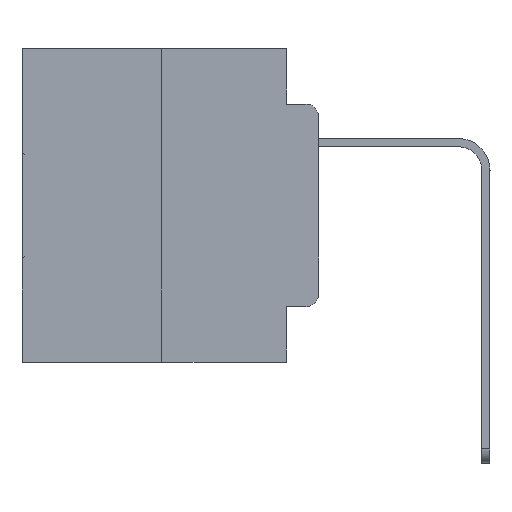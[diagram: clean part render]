
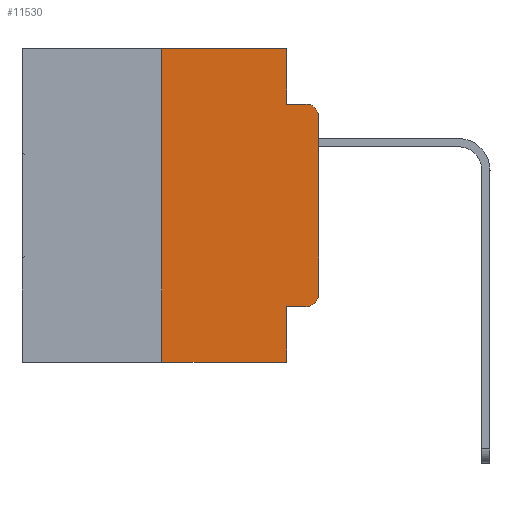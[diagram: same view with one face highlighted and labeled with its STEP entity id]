
A CAD part, left-side view. The second image highlights one B-rep face of the part: STEP entity #11530.
In plain terms, the highlighted planar face has unit normal (-1, 0, 0).
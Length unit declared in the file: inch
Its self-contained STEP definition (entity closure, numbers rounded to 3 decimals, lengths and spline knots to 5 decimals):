
#555 = DIRECTION ( 'NONE',  ( -1., 0., 0. ) ) ;
#612 = ORIENTED_EDGE ( 'NONE', *, *, #26887, .F. ) ;
#956 = CARTESIAN_POINT ( 'NONE',  ( 0., 0.02, -0.4115 ) ) ;
#1612 = LINE ( 'NONE', #6026, #26392 ) ;
#1768 = ORIENTED_EDGE ( 'NONE', *, *, #15779, .T. ) ;
#1941 = VERTEX_POINT ( 'NONE', #22275 ) ;
#2228 = DIRECTION ( 'NONE',  ( -1., 0., 0. ) ) ;
#2858 = CARTESIAN_POINT ( 'NONE',  ( 0., 0.02, -0.3915 ) ) ;
#3165 = DIRECTION ( 'NONE',  ( 0., 0., -1. ) ) ;
#3425 = VECTOR ( 'NONE', #10558, 39.37008 ) ;
#3594 = VERTEX_POINT ( 'NONE', #9480 ) ;
#3764 = DIRECTION ( 'NONE',  ( 0., -1., 0. ) ) ;
#3897 = EDGE_CURVE ( 'NONE', #1941, #20254, #21566, .T. ) ;
#3945 = EDGE_CURVE ( 'NONE', #5392, #29817, #1612, .T. ) ;
#4189 = ORIENTED_EDGE ( 'NONE', *, *, #19723, .T. ) ;
#5392 = VERTEX_POINT ( 'NONE', #6243 ) ;
#5624 = DIRECTION ( 'NONE',  ( 0., -1., 0. ) ) ;
#5630 = LINE ( 'NONE', #12832, #3425 ) ;
#6026 = CARTESIAN_POINT ( 'NONE',  ( 0., 0., 0. ) ) ;
#6243 = CARTESIAN_POINT ( 'NONE',  ( 0., 0., -0.3915 ) ) ;
#6244 = CARTESIAN_POINT ( 'NONE',  ( 0., 0.25, 0. ) ) ;
#7311 = CARTESIAN_POINT ( 'NONE',  ( 0., 0.02, -0.0885 ) ) ;
#8079 = VERTEX_POINT ( 'NONE', #20498 ) ;
#8158 = CARTESIAN_POINT ( 'NONE',  ( 0., 0.051, -0.5 ) ) ;
#8228 = LINE ( 'NONE', #28824, #13765 ) ;
#8421 = VERTEX_POINT ( 'NONE', #7311 ) ;
#9480 = CARTESIAN_POINT ( 'NONE',  ( 0., 0.051, -0.0885 ) ) ;
#10358 = VERTEX_POINT ( 'NONE', #956 ) ;
#10513 = DIRECTION ( 'NONE',  ( 1., 0., 0. ) ) ;
#10558 = DIRECTION ( 'NONE',  ( 0., 0., -1. ) ) ;
#11530 = ADVANCED_FACE ( 'NONE', ( #17773 ), #19885, .F. ) ;
#12347 = ORIENTED_EDGE ( 'NONE', *, *, #20374, .F. ) ;
#12472 = DIRECTION ( 'NONE',  ( 0., -1., 0. ) ) ;
#12832 = CARTESIAN_POINT ( 'NONE',  ( 0., 0.051, 0. ) ) ;
#13064 = LINE ( 'NONE', #17302, #20425 ) ;
#13093 = DIRECTION ( 'NONE',  ( 0., 0., -1. ) ) ;
#13266 = LINE ( 'NONE', #6244, #18780 ) ;
#13474 = DIRECTION ( 'NONE',  ( 0., 0., 1. ) ) ;
#13765 = VECTOR ( 'NONE', #12472, 39.37008 ) ;
#14086 = ORIENTED_EDGE ( 'NONE', *, *, #17543, .T. ) ;
#14752 = DIRECTION ( 'NONE',  ( 0., 0., -1. ) ) ;
#15779 = EDGE_CURVE ( 'NONE', #27083, #28043, #29642, .T. ) ;
#15990 = ORIENTED_EDGE ( 'NONE', *, *, #3897, .F. ) ;
#16454 = CIRCLE ( 'NONE', #26101, 0.02 ) ;
#16767 = CARTESIAN_POINT ( 'NONE',  ( 0., 0.25, -0.5 ) ) ;
#17117 = DIRECTION ( 'NONE',  ( 0., -1., 0. ) ) ;
#17302 = CARTESIAN_POINT ( 'NONE',  ( 0., 0.051, 0. ) ) ;
#17543 = EDGE_CURVE ( 'NONE', #8079, #10358, #19461, .T. ) ;
#17773 = FACE_OUTER_BOUND ( 'NONE', #30167, .T. ) ;
#18365 = VECTOR ( 'NONE', #17117, 39.37008 ) ;
#18780 = VECTOR ( 'NONE', #13474, 39.37008 ) ;
#19461 = LINE ( 'NONE', #28915, #18365 ) ;
#19723 = EDGE_CURVE ( 'NONE', #29817, #8421, #16454, .T. ) ;
#19770 = ORIENTED_EDGE ( 'NONE', *, *, #26565, .T. ) ;
#19861 = VECTOR ( 'NONE', #3764, 39.37008 ) ;
#19885 = PLANE ( 'NONE',  #29152 ) ;
#20029 = CARTESIAN_POINT ( 'NONE',  ( 0., 0.473, -0.5 ) ) ;
#20254 = VERTEX_POINT ( 'NONE', #24049 ) ;
#20291 = CIRCLE ( 'NONE', #28772, 0.02 ) ;
#20374 = EDGE_CURVE ( 'NONE', #8079, #28043, #13064, .T. ) ;
#20425 = VECTOR ( 'NONE', #3165, 39.37008 ) ;
#20498 = CARTESIAN_POINT ( 'NONE',  ( 0., 0.051, -0.4115 ) ) ;
#20572 = DIRECTION ( 'NONE',  ( 0., 0., 1. ) ) ;
#20982 = EDGE_CURVE ( 'NONE', #20254, #3594, #5630, .T. ) ;
#21566 = LINE ( 'NONE', #29088, #23070 ) ;
#22275 = CARTESIAN_POINT ( 'NONE',  ( 0., 0.25, 0. ) ) ;
#23070 = VECTOR ( 'NONE', #5624, 39.37008 ) ;
#23523 = DIRECTION ( 'NONE',  ( 0., 0., -1. ) ) ;
#24049 = CARTESIAN_POINT ( 'NONE',  ( 0., 0.051, 0. ) ) ;
#24660 = ORIENTED_EDGE ( 'NONE', *, *, #24875, .F. ) ;
#24875 = EDGE_CURVE ( 'NONE', #3594, #8421, #8228, .T. ) ;
#25723 = ORIENTED_EDGE ( 'NONE', *, *, #3945, .T. ) ;
#26101 = AXIS2_PLACEMENT_3D ( 'NONE', #30564, #2228, #23523 ) ;
#26302 = CARTESIAN_POINT ( 'NONE',  ( 0., 0., -0.1085 ) ) ;
#26392 = VECTOR ( 'NONE', #20572, 39.37008 ) ;
#26565 = EDGE_CURVE ( 'NONE', #10358, #5392, #20291, .T. ) ;
#26887 = EDGE_CURVE ( 'NONE', #27083, #1941, #13266, .T. ) ;
#27083 = VERTEX_POINT ( 'NONE', #16767 ) ;
#28043 = VERTEX_POINT ( 'NONE', #8158 ) ;
#28772 = AXIS2_PLACEMENT_3D ( 'NONE', #2858, #555, #14752 ) ;
#28824 = CARTESIAN_POINT ( 'NONE',  ( 0., 0.051, -0.0885 ) ) ;
#28915 = CARTESIAN_POINT ( 'NONE',  ( 0., 0.051, -0.4115 ) ) ;
#29082 = ORIENTED_EDGE ( 'NONE', *, *, #20982, .F. ) ;
#29088 = CARTESIAN_POINT ( 'NONE',  ( 0., 0.473, 0. ) ) ;
#29152 = AXIS2_PLACEMENT_3D ( 'NONE', #29540, #10513, #13093 ) ;
#29540 = CARTESIAN_POINT ( 'NONE',  ( 0., 0.473, 0. ) ) ;
#29642 = LINE ( 'NONE', #20029, #19861 ) ;
#29817 = VERTEX_POINT ( 'NONE', #26302 ) ;
#30167 = EDGE_LOOP ( 'NONE', ( #25723, #4189, #24660, #29082, #15990, #612, #1768, #12347, #14086, #19770 ) ) ;
#30564 = CARTESIAN_POINT ( 'NONE',  ( 0., 0.02, -0.1085 ) ) ;
